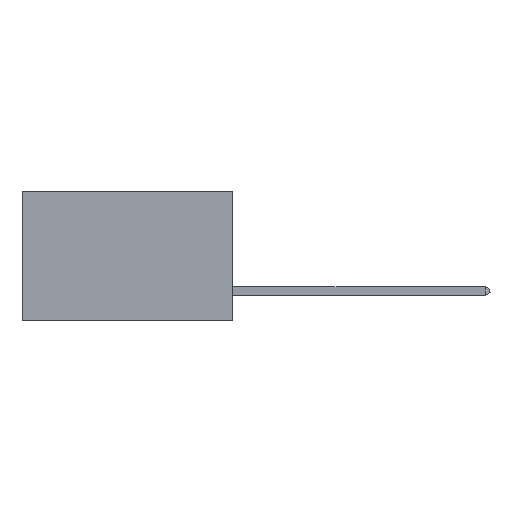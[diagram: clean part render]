
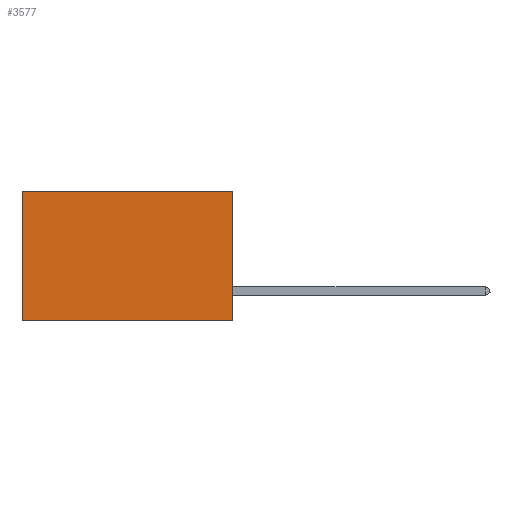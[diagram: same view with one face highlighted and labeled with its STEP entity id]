
A CAD part, left-side view. The second image highlights one B-rep face of the part: STEP entity #3577.
In plain terms, the highlighted planar face has unit normal (-1, 0, 0).
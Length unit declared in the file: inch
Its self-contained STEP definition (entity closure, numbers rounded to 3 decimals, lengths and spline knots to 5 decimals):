
#96 = VERTEX_POINT ( 'NONE', #3212 ) ;
#221 = EDGE_CURVE ( 'NONE', #6581, #4726, #8384, .T. ) ;
#224 = VECTOR ( 'NONE', #7587, 39.37008 ) ;
#460 = EDGE_CURVE ( 'NONE', #96, #2422, #2268, .T. ) ;
#1422 = LINE ( 'NONE', #10679, #4780 ) ;
#2268 = LINE ( 'NONE', #9677, #4996 ) ;
#2343 = VECTOR ( 'NONE', #5354, 39.37008 ) ;
#2422 = VERTEX_POINT ( 'NONE', #10065 ) ;
#2508 = LINE ( 'NONE', #8462, #2343 ) ;
#3151 = FACE_OUTER_BOUND ( 'NONE', #12813, .T. ) ;
#3212 = CARTESIAN_POINT ( 'NONE',  ( 0.2875, 0.6, 0. ) ) ;
#3516 = DIRECTION ( 'NONE',  ( 0., 0., -1. ) ) ;
#3577 = ADVANCED_FACE ( 'NONE', ( #3151 ), #13186, .F. ) ;
#4022 = ORIENTED_EDGE ( 'NONE', *, *, #4500, .F. ) ;
#4023 = CARTESIAN_POINT ( 'NONE',  ( 0.2875, 0., 0. ) ) ;
#4500 = EDGE_CURVE ( 'NONE', #4726, #2422, #1422, .T. ) ;
#4717 = AXIS2_PLACEMENT_3D ( 'NONE', #5996, #13141, #10053 ) ;
#4726 = VERTEX_POINT ( 'NONE', #7784 ) ;
#4780 = VECTOR ( 'NONE', #9785, 39.37008 ) ;
#4996 = VECTOR ( 'NONE', #3516, 39.37008 ) ;
#5354 = DIRECTION ( 'NONE',  ( 0., 1., 0. ) ) ;
#5996 = CARTESIAN_POINT ( 'NONE',  ( 0.2875, 0., 0. ) ) ;
#6581 = VERTEX_POINT ( 'NONE', #9355 ) ;
#7024 = ORIENTED_EDGE ( 'NONE', *, *, #221, .F. ) ;
#7587 = DIRECTION ( 'NONE',  ( 0., 0., -1. ) ) ;
#7784 = CARTESIAN_POINT ( 'NONE',  ( 0.2875, 0., -0.37 ) ) ;
#8384 = LINE ( 'NONE', #4023, #224 ) ;
#8462 = CARTESIAN_POINT ( 'NONE',  ( 0.2875, 0., 0. ) ) ;
#9355 = CARTESIAN_POINT ( 'NONE',  ( 0.2875, 0., 0. ) ) ;
#9677 = CARTESIAN_POINT ( 'NONE',  ( 0.2875, 0.6, 0. ) ) ;
#9785 = DIRECTION ( 'NONE',  ( 0., 1., 0. ) ) ;
#10053 = DIRECTION ( 'NONE',  ( 0., 0., -1. ) ) ;
#10065 = CARTESIAN_POINT ( 'NONE',  ( 0.2875, 0.6, -0.37 ) ) ;
#10278 = EDGE_CURVE ( 'NONE', #6581, #96, #2508, .T. ) ;
#10679 = CARTESIAN_POINT ( 'NONE',  ( 0.2875, 0., -0.37 ) ) ;
#11115 = ORIENTED_EDGE ( 'NONE', *, *, #10278, .T. ) ;
#11664 = ORIENTED_EDGE ( 'NONE', *, *, #460, .T. ) ;
#12813 = EDGE_LOOP ( 'NONE', ( #11664, #4022, #7024, #11115 ) ) ;
#13141 = DIRECTION ( 'NONE',  ( 1., 0., 0. ) ) ;
#13186 = PLANE ( 'NONE',  #4717 ) ;
